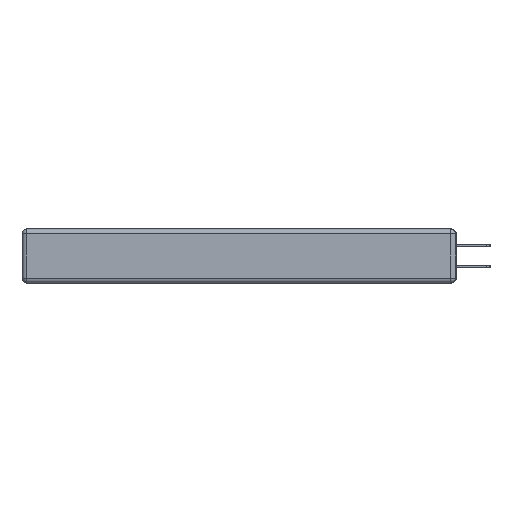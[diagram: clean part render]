
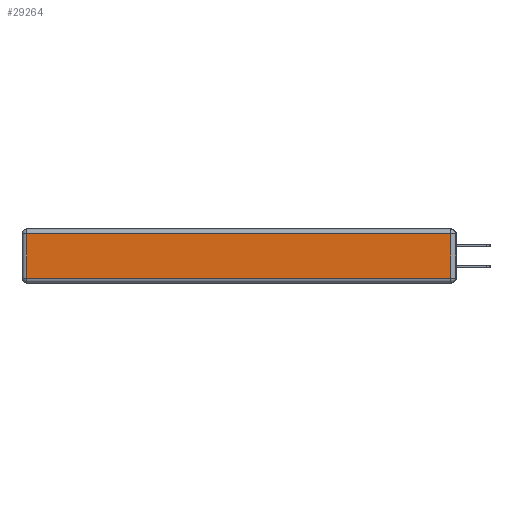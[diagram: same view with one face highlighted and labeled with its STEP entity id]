
A CAD part, left-side view. The second image highlights one B-rep face of the part: STEP entity #29264.
In plain terms, the highlighted planar face has unit normal (-1, 0, 0).
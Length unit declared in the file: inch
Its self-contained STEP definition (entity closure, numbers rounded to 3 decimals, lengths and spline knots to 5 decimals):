
#1130 = LINE ( 'NONE', #7979, #23824 ) ;
#1745 = CARTESIAN_POINT ( 'NONE',  ( 0., 2.72, -0.343 ) ) ;
#2054 = LINE ( 'NONE', #1745, #19357 ) ;
#2238 = ORIENTED_EDGE ( 'NONE', *, *, #4330, .T. ) ;
#4330 = EDGE_CURVE ( 'NONE', #14346, #18989, #2054, .T. ) ;
#6334 = CARTESIAN_POINT ( 'NONE',  ( 0., 2.75, -0.03 ) ) ;
#6747 = DIRECTION ( 'NONE',  ( 0., 1., 0. ) ) ;
#7979 = CARTESIAN_POINT ( 'NONE',  ( 0., 0., -0.313 ) ) ;
#8789 = FACE_OUTER_BOUND ( 'NONE', #17112, .T. ) ;
#9744 = CARTESIAN_POINT ( 'NONE',  ( 0., 2.72, -0.03 ) ) ;
#10166 = ORIENTED_EDGE ( 'NONE', *, *, #21255, .T. ) ;
#10739 = LINE ( 'NONE', #6334, #23006 ) ;
#10794 = AXIS2_PLACEMENT_3D ( 'NONE', #31606, #14586, #29360 ) ;
#11637 = VERTEX_POINT ( 'NONE', #17149 ) ;
#12523 = ORIENTED_EDGE ( 'NONE', *, *, #18653, .T. ) ;
#14346 = VERTEX_POINT ( 'NONE', #9744 ) ;
#14586 = DIRECTION ( 'NONE',  ( -1., 0., 0. ) ) ;
#16488 = DIRECTION ( 'NONE',  ( 0., 0., -1. ) ) ;
#17057 = LINE ( 'NONE', #27131, #20939 ) ;
#17112 = EDGE_LOOP ( 'NONE', ( #21539, #10166, #12523, #2238 ) ) ;
#17149 = CARTESIAN_POINT ( 'NONE',  ( 0., 0.03, -0.03 ) ) ;
#17808 = EDGE_CURVE ( 'NONE', #18989, #25128, #1130, .T. ) ;
#18653 = EDGE_CURVE ( 'NONE', #11637, #14346, #10739, .T. ) ;
#18989 = VERTEX_POINT ( 'NONE', #22463 ) ;
#19357 = VECTOR ( 'NONE', #16488, 39.37008 ) ;
#20161 = CARTESIAN_POINT ( 'NONE',  ( 0., 0.03, -0.313 ) ) ;
#20939 = VECTOR ( 'NONE', #27242, 39.37008 ) ;
#21255 = EDGE_CURVE ( 'NONE', #25128, #11637, #17057, .T. ) ;
#21539 = ORIENTED_EDGE ( 'NONE', *, *, #17808, .T. ) ;
#22463 = CARTESIAN_POINT ( 'NONE',  ( 0., 2.72, -0.313 ) ) ;
#23006 = VECTOR ( 'NONE', #6747, 39.37008 ) ;
#23824 = VECTOR ( 'NONE', #30081, 39.37008 ) ;
#25128 = VERTEX_POINT ( 'NONE', #20161 ) ;
#27131 = CARTESIAN_POINT ( 'NONE',  ( 0., 0.03, -0.343 ) ) ;
#27242 = DIRECTION ( 'NONE',  ( 0., 0., 1. ) ) ;
#29264 = ADVANCED_FACE ( 'NONE', ( #8789 ), #31712, .T. ) ;
#29360 = DIRECTION ( 'NONE',  ( 0., 0., 1. ) ) ;
#30081 = DIRECTION ( 'NONE',  ( 0., -1., 0. ) ) ;
#31606 = CARTESIAN_POINT ( 'NONE',  ( 0., 0., -0.343 ) ) ;
#31712 = PLANE ( 'NONE',  #10794 ) ;
